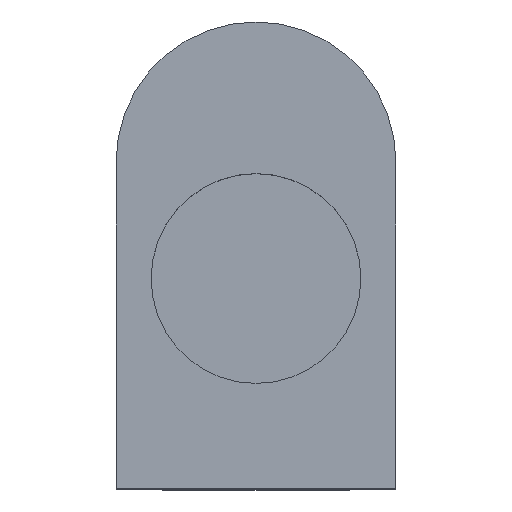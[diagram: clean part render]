
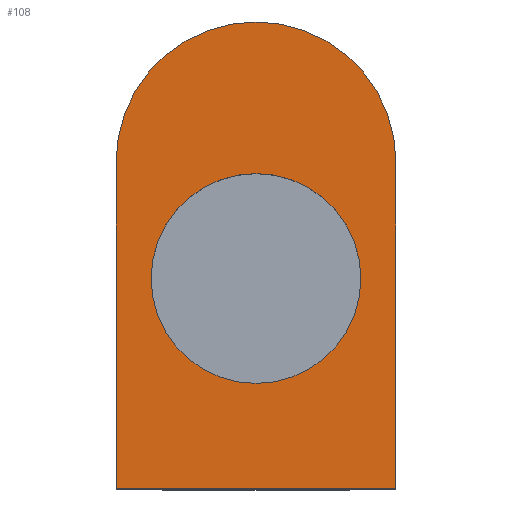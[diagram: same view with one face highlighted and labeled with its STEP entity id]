
A CAD part, top view. The second image highlights one B-rep face of the part: STEP entity #108.
In plain terms, the highlighted planar face has unit normal (0, 0, 1).
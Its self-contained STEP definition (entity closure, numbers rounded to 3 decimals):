
#1 = EDGE_LOOP ( 'NONE', ( #276, #262, #173, #490 ) ) ;
#18 = CARTESIAN_POINT ( 'NONE',  ( 6., -14., 40. ) ) ;
#36 = AXIS2_PLACEMENT_3D ( 'NONE', #384, #708, #316 ) ;
#81 = EDGE_CURVE ( 'NONE', #756, #674, #642, .T. ) ;
#108 = ADVANCED_FACE ( 'NONE', ( #824, #254 ), #842, .T. ) ;
#139 = ORIENTED_EDGE ( 'NONE', *, *, #151, .T. ) ;
#151 = EDGE_CURVE ( 'NONE', #273, #570, #533, .T. ) ;
#161 = DIRECTION ( 'NONE',  ( 1., 0., 0. ) ) ;
#173 = ORIENTED_EDGE ( 'NONE', *, *, #416, .T. ) ;
#188 = CARTESIAN_POINT ( 'NONE',  ( 0., -5., 40. ) ) ;
#193 = CIRCLE ( 'NONE', #521, 4.5 ) ;
#205 = LINE ( 'NONE', #18, #293 ) ;
#210 = CARTESIAN_POINT ( 'NONE',  ( 6., 0., 40. ) ) ;
#229 = LINE ( 'NONE', #491, #499 ) ;
#254 = FACE_OUTER_BOUND ( 'NONE', #1, .T. ) ;
#258 = DIRECTION ( 'NONE',  ( 1., 0., 0. ) ) ;
#262 = ORIENTED_EDGE ( 'NONE', *, *, #495, .T. ) ;
#273 = VERTEX_POINT ( 'NONE', #274 ) ;
#274 = CARTESIAN_POINT ( 'NONE',  ( 4.5, -5., 40. ) ) ;
#276 = ORIENTED_EDGE ( 'NONE', *, *, #81, .T. ) ;
#283 = AXIS2_PLACEMENT_3D ( 'NONE', #518, #380, #258 ) ;
#293 = VECTOR ( 'NONE', #788, 1000. ) ;
#299 = EDGE_CURVE ( 'NONE', #632, #756, #205, .T. ) ;
#308 = CARTESIAN_POINT ( 'NONE',  ( -6., 0., 40. ) ) ;
#316 = DIRECTION ( 'NONE',  ( 1., 0., 0. ) ) ;
#338 = DIRECTION ( 'NONE',  ( 0., 0., -1. ) ) ;
#380 = DIRECTION ( 'NONE',  ( 0., 0., 1. ) ) ;
#384 = CARTESIAN_POINT ( 'NONE',  ( 0., 0., 40. ) ) ;
#416 = EDGE_CURVE ( 'NONE', #741, #632, #229, .T. ) ;
#455 = DIRECTION ( 'NONE',  ( 1., 0., 0. ) ) ;
#456 = CARTESIAN_POINT ( 'NONE',  ( 6., -14., 40. ) ) ;
#472 = ORIENTED_EDGE ( 'NONE', *, *, #733, .T. ) ;
#490 = ORIENTED_EDGE ( 'NONE', *, *, #299, .T. ) ;
#491 = CARTESIAN_POINT ( 'NONE',  ( -6., -14., 40. ) ) ;
#495 = EDGE_CURVE ( 'NONE', #674, #741, #577, .T. ) ;
#499 = VECTOR ( 'NONE', #161, 1000. ) ;
#509 = CARTESIAN_POINT ( 'NONE',  ( -4.5, -5., 40. ) ) ;
#518 = CARTESIAN_POINT ( 'NONE',  ( 0., 0., 40. ) ) ;
#521 = AXIS2_PLACEMENT_3D ( 'NONE', #801, #338, #735 ) ;
#533 = CIRCLE ( 'NONE', #804, 4.5 ) ;
#542 = VECTOR ( 'NONE', #838, 1000. ) ;
#570 = VERTEX_POINT ( 'NONE', #509 ) ;
#577 = LINE ( 'NONE', #580, #542 ) ;
#580 = CARTESIAN_POINT ( 'NONE',  ( -6., 0., 40. ) ) ;
#632 = VERTEX_POINT ( 'NONE', #456 ) ;
#642 = CIRCLE ( 'NONE', #36, 6. ) ;
#652 = DIRECTION ( 'NONE',  ( 0., 0., -1. ) ) ;
#674 = VERTEX_POINT ( 'NONE', #308 ) ;
#708 = DIRECTION ( 'NONE',  ( 0., 0., 1. ) ) ;
#718 = CARTESIAN_POINT ( 'NONE',  ( -6., -14., 40. ) ) ;
#722 = EDGE_LOOP ( 'NONE', ( #472, #139 ) ) ;
#733 = EDGE_CURVE ( 'NONE', #570, #273, #193, .T. ) ;
#735 = DIRECTION ( 'NONE',  ( 1., 0., 0. ) ) ;
#741 = VERTEX_POINT ( 'NONE', #718 ) ;
#756 = VERTEX_POINT ( 'NONE', #210 ) ;
#788 = DIRECTION ( 'NONE',  ( 0., 1., 0. ) ) ;
#801 = CARTESIAN_POINT ( 'NONE',  ( 0., -5., 40. ) ) ;
#804 = AXIS2_PLACEMENT_3D ( 'NONE', #188, #652, #455 ) ;
#824 = FACE_BOUND ( 'NONE', #722, .T. ) ;
#838 = DIRECTION ( 'NONE',  ( 0., -1., 0. ) ) ;
#842 = PLANE ( 'NONE',  #283 ) ;
